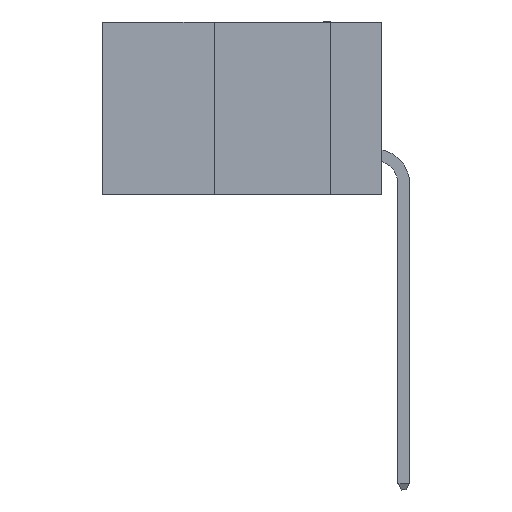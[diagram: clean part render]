
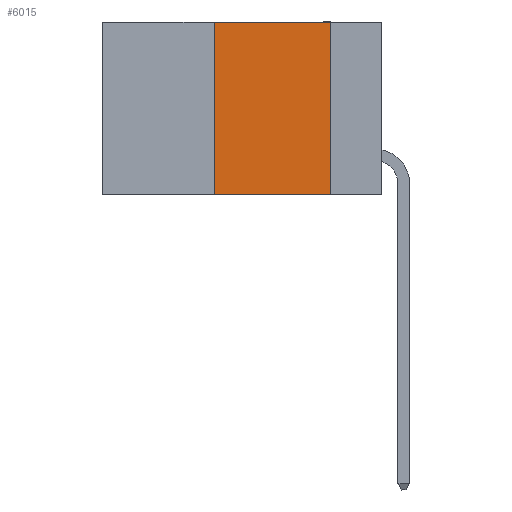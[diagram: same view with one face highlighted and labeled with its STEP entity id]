
A CAD part, left-side view. The second image highlights one B-rep face of the part: STEP entity #6015.
In plain terms, the highlighted planar face has unit normal (-1, 0, 0).
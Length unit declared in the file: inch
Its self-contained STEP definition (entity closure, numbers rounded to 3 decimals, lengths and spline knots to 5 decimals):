
#614 = EDGE_CURVE ( 'NONE', #24863, #2770, #20803, .T. ) ;
#731 = VECTOR ( 'NONE', #24410, 39.37008 ) ;
#1687 = EDGE_CURVE ( 'NONE', #7458, #35574, #16041, .T. ) ;
#2770 = VERTEX_POINT ( 'NONE', #27788 ) ;
#5783 = ORIENTED_EDGE ( 'NONE', *, *, #614, .F. ) ;
#6015 = ADVANCED_FACE ( 'NONE', ( #14136 ), #12240, .F. ) ;
#6649 = DIRECTION ( 'NONE',  ( 1., 0., 0. ) ) ;
#7016 = EDGE_CURVE ( 'NONE', #35574, #24863, #25305, .T. ) ;
#7458 = VERTEX_POINT ( 'NONE', #36378 ) ;
#9412 = VECTOR ( 'NONE', #10916, 39.37008 ) ;
#10005 = EDGE_LOOP ( 'NONE', ( #5783, #30932, #17566, #14137 ) ) ;
#10916 = DIRECTION ( 'NONE',  ( 0., 0., 1. ) ) ;
#11572 = DIRECTION ( 'NONE',  ( 0., -1., 0. ) ) ;
#12240 = PLANE ( 'NONE',  #32492 ) ;
#12611 = VECTOR ( 'NONE', #40653, 39.37008 ) ;
#13936 = CARTESIAN_POINT ( 'NONE',  ( 0., 0.11, 0. ) ) ;
#14111 = CARTESIAN_POINT ( 'NONE',  ( 0., 0.6, 0. ) ) ;
#14136 = FACE_OUTER_BOUND ( 'NONE', #10005, .T. ) ;
#14137 = ORIENTED_EDGE ( 'NONE', *, *, #29348, .T. ) ;
#16041 = LINE ( 'NONE', #30501, #9412 ) ;
#17566 = ORIENTED_EDGE ( 'NONE', *, *, #1687, .F. ) ;
#20803 = LINE ( 'NONE', #13936, #12611 ) ;
#23772 = CARTESIAN_POINT ( 'NONE',  ( 0., 0.36, 0. ) ) ;
#24410 = DIRECTION ( 'NONE',  ( 0., -1., 0. ) ) ;
#24863 = VERTEX_POINT ( 'NONE', #30854 ) ;
#25305 = LINE ( 'NONE', #14111, #731 ) ;
#26506 = CARTESIAN_POINT ( 'NONE',  ( 0., 0.6, 0. ) ) ;
#26863 = VECTOR ( 'NONE', #11572, 39.37008 ) ;
#27788 = CARTESIAN_POINT ( 'NONE',  ( 0., 0.11, -0.37 ) ) ;
#28047 = LINE ( 'NONE', #31158, #26863 ) ;
#29348 = EDGE_CURVE ( 'NONE', #7458, #2770, #28047, .T. ) ;
#30501 = CARTESIAN_POINT ( 'NONE',  ( 0., 0.36, 0. ) ) ;
#30854 = CARTESIAN_POINT ( 'NONE',  ( 0., 0.11, 0. ) ) ;
#30932 = ORIENTED_EDGE ( 'NONE', *, *, #7016, .F. ) ;
#31158 = CARTESIAN_POINT ( 'NONE',  ( 0., 0.6, -0.37 ) ) ;
#32492 = AXIS2_PLACEMENT_3D ( 'NONE', #26506, #6649, #39195 ) ;
#35574 = VERTEX_POINT ( 'NONE', #23772 ) ;
#36378 = CARTESIAN_POINT ( 'NONE',  ( 0., 0.36, -0.37 ) ) ;
#39195 = DIRECTION ( 'NONE',  ( 0., 0., -1. ) ) ;
#40653 = DIRECTION ( 'NONE',  ( 0., 0., -1. ) ) ;
